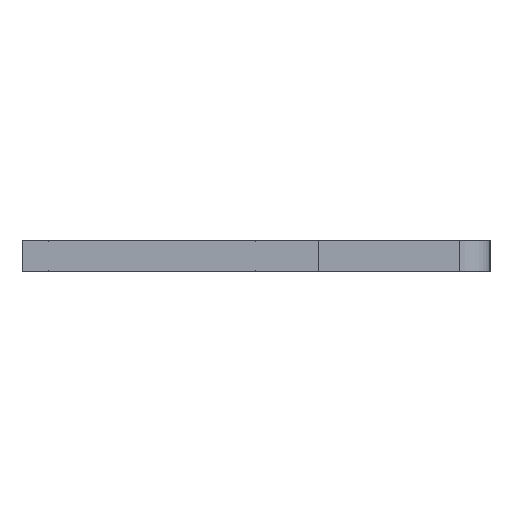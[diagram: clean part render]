
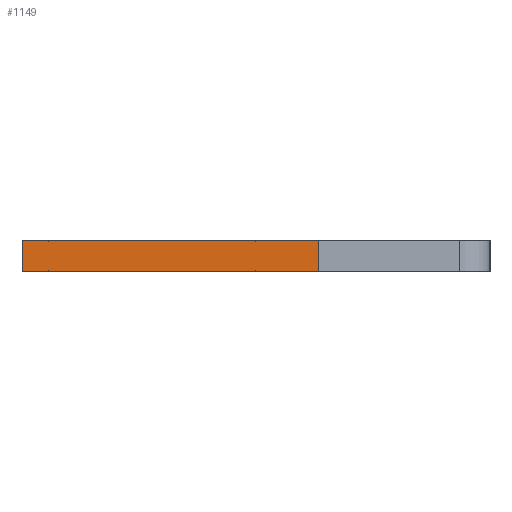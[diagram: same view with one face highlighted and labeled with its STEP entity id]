
A CAD part, left-side view. The second image highlights one B-rep face of the part: STEP entity #1149.
In plain terms, the highlighted face is planar.
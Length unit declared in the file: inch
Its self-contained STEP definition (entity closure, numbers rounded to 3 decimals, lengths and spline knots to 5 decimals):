
#19 = ORIENTED_EDGE ( 'NONE', *, *, #430, .F. ) ;
#78 = AXIS2_PLACEMENT_3D ( 'NONE', #874, #592, #89 ) ;
#89 = DIRECTION ( 'NONE',  ( 1., 0., 0. ) ) ;
#260 = PLANE ( 'NONE',  #78 ) ;
#264 = CARTESIAN_POINT ( 'NONE',  ( 0.01, -0.04, -0.04 ) ) ;
#316 = VECTOR ( 'NONE', #1094, 39.37008 ) ;
#334 = VERTEX_POINT ( 'NONE', #1300 ) ;
#430 = EDGE_CURVE ( 'NONE', #1294, #1550, #1874, .T. ) ;
#445 = CARTESIAN_POINT ( 'NONE',  ( -0.01, 0.15, -0.04 ) ) ;
#467 = EDGE_CURVE ( 'NONE', #1294, #334, #639, .T. ) ;
#592 = DIRECTION ( 'NONE',  ( 0., 0., 1. ) ) ;
#639 = LINE ( 'NONE', #1935, #837 ) ;
#679 = DIRECTION ( 'NONE',  ( 0., 1., 0. ) ) ;
#837 = VECTOR ( 'NONE', #1619, 39.37008 ) ;
#874 = CARTESIAN_POINT ( 'NONE',  ( 0.01, 0.15, -0.04 ) ) ;
#968 = VECTOR ( 'NONE', #679, 39.37008 ) ;
#1051 = LINE ( 'NONE', #1719, #316 ) ;
#1094 = DIRECTION ( 'NONE',  ( -1., 0., 0. ) ) ;
#1147 = LINE ( 'NONE', #2017, #1604 ) ;
#1149 = ADVANCED_FACE ( 'NONE', ( #1656 ), #260, .F. ) ;
#1290 = ORIENTED_EDGE ( 'NONE', *, *, #1521, .F. ) ;
#1294 = VERTEX_POINT ( 'NONE', #264 ) ;
#1300 = CARTESIAN_POINT ( 'NONE',  ( -0.01, -0.04, -0.04 ) ) ;
#1301 = EDGE_CURVE ( 'NONE', #334, #1501, #1147, .T. ) ;
#1501 = VERTEX_POINT ( 'NONE', #445 ) ;
#1521 = EDGE_CURVE ( 'NONE', #1550, #1501, #1051, .T. ) ;
#1550 = VERTEX_POINT ( 'NONE', #1878 ) ;
#1604 = VECTOR ( 'NONE', #1857, 39.37008 ) ;
#1619 = DIRECTION ( 'NONE',  ( -1., 0., 0. ) ) ;
#1627 = CARTESIAN_POINT ( 'NONE',  ( 0.01, 0.15, -0.04 ) ) ;
#1656 = FACE_OUTER_BOUND ( 'NONE', #1931, .T. ) ;
#1719 = CARTESIAN_POINT ( 'NONE',  ( 0.01, 0.15, -0.04 ) ) ;
#1741 = ORIENTED_EDGE ( 'NONE', *, *, #1301, .T. ) ;
#1822 = ORIENTED_EDGE ( 'NONE', *, *, #467, .T. ) ;
#1857 = DIRECTION ( 'NONE',  ( 0., 1., 0. ) ) ;
#1874 = LINE ( 'NONE', #1627, #968 ) ;
#1878 = CARTESIAN_POINT ( 'NONE',  ( 0.01, 0.15, -0.04 ) ) ;
#1931 = EDGE_LOOP ( 'NONE', ( #1741, #1290, #19, #1822 ) ) ;
#1935 = CARTESIAN_POINT ( 'NONE',  ( 0.01, -0.04, -0.04 ) ) ;
#2017 = CARTESIAN_POINT ( 'NONE',  ( -0.01, 0.15, -0.04 ) ) ;
